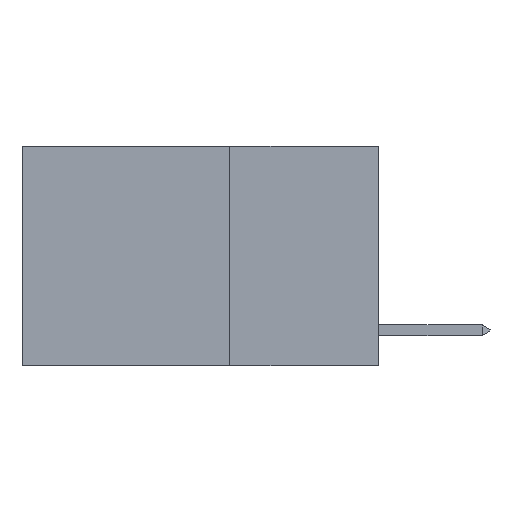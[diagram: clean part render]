
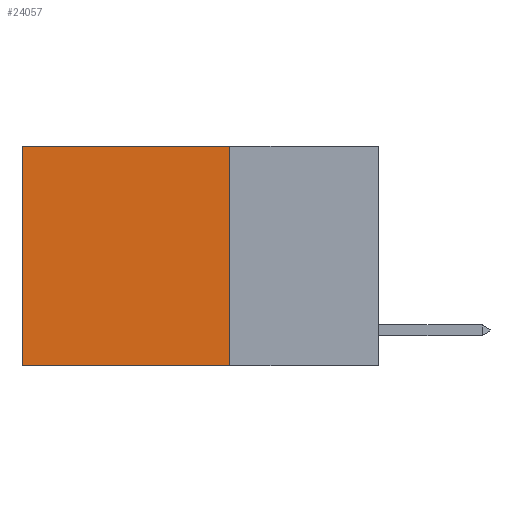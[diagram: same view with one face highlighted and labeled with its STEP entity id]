
A CAD part, left-side view. The second image highlights one B-rep face of the part: STEP entity #24057.
In plain terms, the highlighted planar face has unit normal (-1, 0, 0).
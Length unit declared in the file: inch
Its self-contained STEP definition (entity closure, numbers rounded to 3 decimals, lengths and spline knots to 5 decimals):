
#328 = ORIENTED_EDGE ( 'NONE', *, *, #19854, .F. ) ;
#334 = CARTESIAN_POINT ( 'NONE',  ( 0.2625, 0.25, 0. ) ) ;
#346 = DIRECTION ( 'NONE',  ( 1., 0., 0. ) ) ;
#1631 = CARTESIAN_POINT ( 'NONE',  ( 0.2625, 0.25, 0. ) ) ;
#2176 = VECTOR ( 'NONE', #23644, 39.37008 ) ;
#2601 = DIRECTION ( 'NONE',  ( 0., 0., -1. ) ) ;
#5879 = VERTEX_POINT ( 'NONE', #13596 ) ;
#6440 = LINE ( 'NONE', #334, #22237 ) ;
#9838 = EDGE_CURVE ( 'NONE', #23534, #19635, #6440, .T. ) ;
#11493 = AXIS2_PLACEMENT_3D ( 'NONE', #14948, #346, #2601 ) ;
#11735 = LINE ( 'NONE', #1631, #16225 ) ;
#12697 = PLANE ( 'NONE',  #11493 ) ;
#13457 = ORIENTED_EDGE ( 'NONE', *, *, #25644, .F. ) ;
#13596 = CARTESIAN_POINT ( 'NONE',  ( 0.2625, 0.6, -0.37 ) ) ;
#14948 = CARTESIAN_POINT ( 'NONE',  ( 0.2625, 0.25, 0. ) ) ;
#15056 = LINE ( 'NONE', #25501, #2176 ) ;
#15284 = VERTEX_POINT ( 'NONE', #21309 ) ;
#15718 = DIRECTION ( 'NONE',  ( 0., 0., -1. ) ) ;
#16225 = VECTOR ( 'NONE', #15718, 39.37008 ) ;
#16430 = DIRECTION ( 'NONE',  ( 0., 0., -1. ) ) ;
#16845 = CARTESIAN_POINT ( 'NONE',  ( 0.2625, 0.25, 0. ) ) ;
#19525 = ORIENTED_EDGE ( 'NONE', *, *, #9838, .T. ) ;
#19635 = VERTEX_POINT ( 'NONE', #19979 ) ;
#19640 = EDGE_LOOP ( 'NONE', ( #23175, #328, #13457, #19525 ) ) ;
#19854 = EDGE_CURVE ( 'NONE', #15284, #5879, #15056, .T. ) ;
#19979 = CARTESIAN_POINT ( 'NONE',  ( 0.2625, 0.6, 0. ) ) ;
#20357 = VECTOR ( 'NONE', #16430, 39.37008 ) ;
#20365 = DIRECTION ( 'NONE',  ( 0., 1., 0. ) ) ;
#21309 = CARTESIAN_POINT ( 'NONE',  ( 0.2625, 0.25, -0.37 ) ) ;
#22108 = LINE ( 'NONE', #22491, #20357 ) ;
#22237 = VECTOR ( 'NONE', #20365, 39.37008 ) ;
#22491 = CARTESIAN_POINT ( 'NONE',  ( 0.2625, 0.6, 0. ) ) ;
#23175 = ORIENTED_EDGE ( 'NONE', *, *, #23913, .T. ) ;
#23534 = VERTEX_POINT ( 'NONE', #16845 ) ;
#23644 = DIRECTION ( 'NONE',  ( 0., 1., 0. ) ) ;
#23913 = EDGE_CURVE ( 'NONE', #19635, #5879, #22108, .T. ) ;
#24057 = ADVANCED_FACE ( 'NONE', ( #24999 ), #12697, .F. ) ;
#24999 = FACE_OUTER_BOUND ( 'NONE', #19640, .T. ) ;
#25501 = CARTESIAN_POINT ( 'NONE',  ( 0.2625, 0.25, -0.37 ) ) ;
#25644 = EDGE_CURVE ( 'NONE', #23534, #15284, #11735, .T. ) ;
